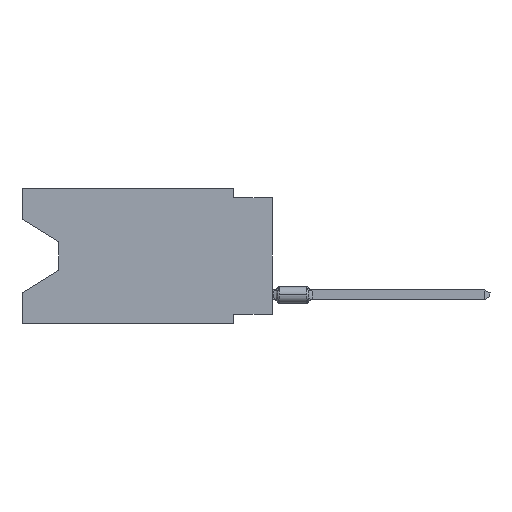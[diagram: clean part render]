
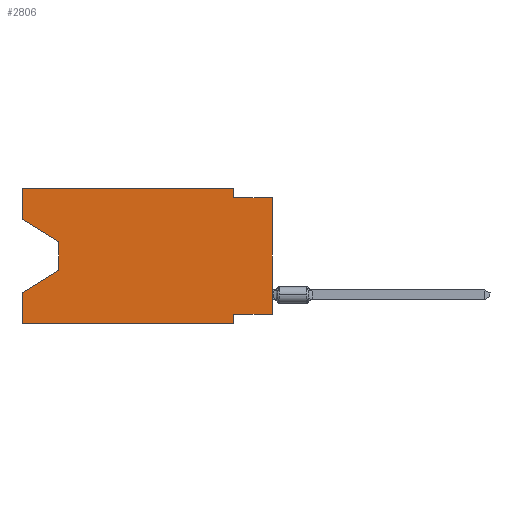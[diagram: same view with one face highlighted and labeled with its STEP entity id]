
A CAD part, left-side view. The second image highlights one B-rep face of the part: STEP entity #2806.
In plain terms, the highlighted planar face has unit normal (-1, 0, 0).
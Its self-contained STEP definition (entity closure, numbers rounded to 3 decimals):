
#291 = EDGE_CURVE ( 'NONE', #12926, #54585, #34481, .T. ) ;
#1009 = LINE ( 'NONE', #27523, #52365 ) ;
#1428 = CARTESIAN_POINT ( 'NONE',  ( 0., 13.97, -5.385 ) ) ;
#1583 = EDGE_LOOP ( 'NONE', ( #11175, #46112, #2476, #22297, #24916, #8888, #32513, #6811, #46455, #41584, #19895, #30561 ) ) ;
#1939 = VERTEX_POINT ( 'NONE', #16170 ) ;
#2476 = ORIENTED_EDGE ( 'NONE', *, *, #44291, .T. ) ;
#2776 = DIRECTION ( 'NONE',  ( 0., 0., -1. ) ) ;
#2806 = ADVANCED_FACE ( 'NONE', ( #38229 ), #34007, .F. ) ;
#3114 = CARTESIAN_POINT ( 'NONE',  ( 0., 0., -0.635 ) ) ;
#3878 = LINE ( 'NONE', #37706, #23038 ) ;
#4113 = DIRECTION ( 'NONE',  ( 0., 0., -1. ) ) ;
#4172 = EDGE_CURVE ( 'NONE', #15483, #1939, #41695, .T. ) ;
#4372 = CARTESIAN_POINT ( 'NONE',  ( 0., 0., -8.255 ) ) ;
#5470 = EDGE_CURVE ( 'NONE', #1939, #51058, #40116, .T. ) ;
#6310 = VECTOR ( 'NONE', #6988, 1000. ) ;
#6810 = CARTESIAN_POINT ( 'NONE',  ( 0., 16.383, -6.852 ) ) ;
#6811 = ORIENTED_EDGE ( 'NONE', *, *, #48052, .T. ) ;
#6988 = DIRECTION ( 'NONE',  ( 0., -0.855, -0.519 ) ) ;
#8888 = ORIENTED_EDGE ( 'NONE', *, *, #9358, .F. ) ;
#9358 = EDGE_CURVE ( 'NONE', #10091, #29147, #3878, .T. ) ;
#9902 = CARTESIAN_POINT ( 'NONE',  ( 0., 16.383, 0. ) ) ;
#10091 = VERTEX_POINT ( 'NONE', #49860 ) ;
#10911 = VECTOR ( 'NONE', #51440, 1000. ) ;
#11000 = VERTEX_POINT ( 'NONE', #23168 ) ;
#11175 = ORIENTED_EDGE ( 'NONE', *, *, #22534, .T. ) ;
#12582 = CARTESIAN_POINT ( 'NONE',  ( 0., 16.383, 0. ) ) ;
#12926 = VERTEX_POINT ( 'NONE', #30107 ) ;
#13923 = VECTOR ( 'NONE', #15897, 1000. ) ;
#15483 = VERTEX_POINT ( 'NONE', #31477 ) ;
#15897 = DIRECTION ( 'NONE',  ( 0., 0.855, -0.519 ) ) ;
#16028 = DIRECTION ( 'NONE',  ( 0., 0., -1. ) ) ;
#16170 = CARTESIAN_POINT ( 'NONE',  ( 0., 2.54, 0. ) ) ;
#17368 = LINE ( 'NONE', #39043, #28544 ) ;
#17550 = LINE ( 'NONE', #9902, #31639 ) ;
#18504 = DIRECTION ( 'NONE',  ( 0., 1., 0. ) ) ;
#19895 = ORIENTED_EDGE ( 'NONE', *, *, #4172, .F. ) ;
#20591 = CARTESIAN_POINT ( 'NONE',  ( 0., 16.383, 0. ) ) ;
#21000 = CARTESIAN_POINT ( 'NONE',  ( 0., 16.383, 0. ) ) ;
#21857 = CARTESIAN_POINT ( 'NONE',  ( 0., 16.383, -8.89 ) ) ;
#22297 = ORIENTED_EDGE ( 'NONE', *, *, #291, .F. ) ;
#22534 = EDGE_CURVE ( 'NONE', #52901, #11000, #55192, .T. ) ;
#23038 = VECTOR ( 'NONE', #2776, 1000. ) ;
#23168 = CARTESIAN_POINT ( 'NONE',  ( 0., 13.97, -3.505 ) ) ;
#23535 = CARTESIAN_POINT ( 'NONE',  ( 0., 0., -0.635 ) ) ;
#23755 = EDGE_CURVE ( 'NONE', #52901, #15483, #17550, .T. ) ;
#24260 = DIRECTION ( 'NONE',  ( 0., -1., 0. ) ) ;
#24356 = LINE ( 'NONE', #41518, #51104 ) ;
#24578 = VECTOR ( 'NONE', #24260, 1000. ) ;
#24916 = ORIENTED_EDGE ( 'NONE', *, *, #50927, .T. ) ;
#27523 = CARTESIAN_POINT ( 'NONE',  ( 0., 0., -8.255 ) ) ;
#28544 = VECTOR ( 'NONE', #16028, 1000. ) ;
#29147 = VERTEX_POINT ( 'NONE', #37623 ) ;
#29918 = EDGE_CURVE ( 'NONE', #38010, #10091, #1009, .T. ) ;
#30107 = CARTESIAN_POINT ( 'NONE',  ( 0., 16.383, -8.89 ) ) ;
#30561 = ORIENTED_EDGE ( 'NONE', *, *, #23755, .F. ) ;
#30915 = VECTOR ( 'NONE', #48868, 1000. ) ;
#31142 = CARTESIAN_POINT ( 'NONE',  ( 0., 16.383, -2.038 ) ) ;
#31477 = CARTESIAN_POINT ( 'NONE',  ( 0., 16.383, 0. ) ) ;
#31639 = VECTOR ( 'NONE', #52216, 1000. ) ;
#32066 = VERTEX_POINT ( 'NONE', #1428 ) ;
#32513 = ORIENTED_EDGE ( 'NONE', *, *, #29918, .F. ) ;
#34007 = PLANE ( 'NONE',  #39491 ) ;
#34481 = LINE ( 'NONE', #21000, #53803 ) ;
#35061 = LINE ( 'NONE', #21857, #10911 ) ;
#37310 = CARTESIAN_POINT ( 'NONE',  ( 0., 13.97, -5.385 ) ) ;
#37623 = CARTESIAN_POINT ( 'NONE',  ( 0., 2.54, -8.89 ) ) ;
#37706 = CARTESIAN_POINT ( 'NONE',  ( 0., 2.54, -8.89 ) ) ;
#37869 = LINE ( 'NONE', #37310, #13923 ) ;
#38010 = VERTEX_POINT ( 'NONE', #4372 ) ;
#38229 = FACE_OUTER_BOUND ( 'NONE', #1583, .T. ) ;
#39043 = CARTESIAN_POINT ( 'NONE',  ( 0., 13.97, -3.505 ) ) ;
#39491 = AXIS2_PLACEMENT_3D ( 'NONE', #12582, #42730, #4113 ) ;
#40116 = LINE ( 'NONE', #49716, #30915 ) ;
#40686 = CARTESIAN_POINT ( 'NONE',  ( 0., 2.54, -0.635 ) ) ;
#41518 = CARTESIAN_POINT ( 'NONE',  ( 0., 0., 0. ) ) ;
#41584 = ORIENTED_EDGE ( 'NONE', *, *, #5470, .F. ) ;
#41695 = LINE ( 'NONE', #20591, #24578 ) ;
#41731 = LINE ( 'NONE', #3114, #52336 ) ;
#42730 = DIRECTION ( 'NONE',  ( 1., 0., 0. ) ) ;
#43781 = DIRECTION ( 'NONE',  ( 0., -1., 0. ) ) ;
#44291 = EDGE_CURVE ( 'NONE', #32066, #54585, #37869, .T. ) ;
#45616 = CARTESIAN_POINT ( 'NONE',  ( 0., 16.383, -2.038 ) ) ;
#46112 = ORIENTED_EDGE ( 'NONE', *, *, #46772, .T. ) ;
#46455 = ORIENTED_EDGE ( 'NONE', *, *, #50833, .F. ) ;
#46772 = EDGE_CURVE ( 'NONE', #11000, #32066, #17368, .T. ) ;
#48052 = EDGE_CURVE ( 'NONE', #38010, #51066, #24356, .T. ) ;
#48868 = DIRECTION ( 'NONE',  ( 0., 0., -1. ) ) ;
#49716 = CARTESIAN_POINT ( 'NONE',  ( 0., 2.54, 0. ) ) ;
#49860 = CARTESIAN_POINT ( 'NONE',  ( 0., 2.54, -8.255 ) ) ;
#50270 = DIRECTION ( 'NONE',  ( 0., 0., 1. ) ) ;
#50833 = EDGE_CURVE ( 'NONE', #51058, #51066, #41731, .T. ) ;
#50927 = EDGE_CURVE ( 'NONE', #12926, #29147, #35061, .T. ) ;
#51058 = VERTEX_POINT ( 'NONE', #40686 ) ;
#51066 = VERTEX_POINT ( 'NONE', #23535 ) ;
#51104 = VECTOR ( 'NONE', #50270, 1000. ) ;
#51440 = DIRECTION ( 'NONE',  ( 0., -1., 0. ) ) ;
#51686 = DIRECTION ( 'NONE',  ( 0., 0., 1. ) ) ;
#52216 = DIRECTION ( 'NONE',  ( 0., 0., 1. ) ) ;
#52336 = VECTOR ( 'NONE', #43781, 1000. ) ;
#52365 = VECTOR ( 'NONE', #18504, 1000. ) ;
#52901 = VERTEX_POINT ( 'NONE', #31142 ) ;
#53803 = VECTOR ( 'NONE', #51686, 1000. ) ;
#54585 = VERTEX_POINT ( 'NONE', #6810 ) ;
#55192 = LINE ( 'NONE', #45616, #6310 ) ;
